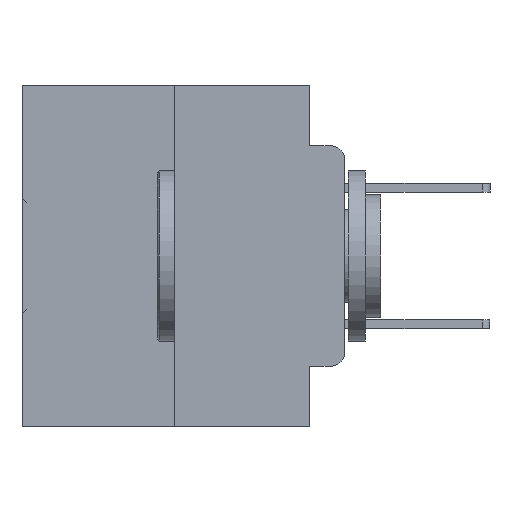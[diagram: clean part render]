
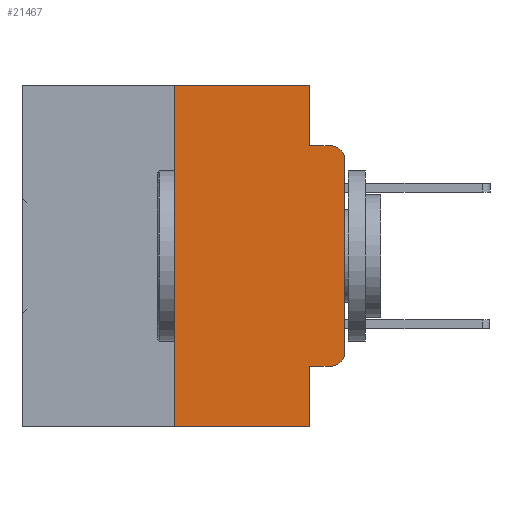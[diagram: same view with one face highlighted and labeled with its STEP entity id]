
A CAD part, left-side view. The second image highlights one B-rep face of the part: STEP entity #21467.
In plain terms, the highlighted planar face has unit normal (-1, 0, 0).
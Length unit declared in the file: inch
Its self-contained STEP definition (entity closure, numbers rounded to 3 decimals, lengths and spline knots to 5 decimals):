
#123 = EDGE_CURVE ( 'NONE', #16070, #5999, #28364, .T. ) ;
#210 = AXIS2_PLACEMENT_3D ( 'NONE', #16920, #19597, #10904 ) ;
#654 = DIRECTION ( 'NONE',  ( 0., 0., 1. ) ) ;
#675 = AXIS2_PLACEMENT_3D ( 'NONE', #14269, #32561, #16917 ) ;
#773 = AXIS2_PLACEMENT_3D ( 'NONE', #9756, #28203, #12435 ) ;
#1258 = EDGE_CURVE ( 'NONE', #7230, #16070, #28682, .T. ) ;
#2096 = DIRECTION ( 'NONE',  ( 0., -1., 0. ) ) ;
#2552 = DIRECTION ( 'NONE',  ( 0., 0., -1. ) ) ;
#2671 = CARTESIAN_POINT ( 'NONE',  ( 0., 0.051, -0.5 ) ) ;
#2820 = DIRECTION ( 'NONE',  ( 0., 0., 1. ) ) ;
#3560 = DIRECTION ( 'NONE',  ( 0., -1., 0. ) ) ;
#3790 = CARTESIAN_POINT ( 'NONE',  ( 0., 0.051, -0.0885 ) ) ;
#5045 = ORIENTED_EDGE ( 'NONE', *, *, #31380, .F. ) ;
#5073 = DIRECTION ( 'NONE',  ( 0., -1., 0. ) ) ;
#5190 = EDGE_CURVE ( 'NONE', #10859, #33024, #15728, .T. ) ;
#5338 = CARTESIAN_POINT ( 'NONE',  ( 0., 0., -0.3915 ) ) ;
#5439 = VERTEX_POINT ( 'NONE', #19984 ) ;
#5999 = VERTEX_POINT ( 'NONE', #5338 ) ;
#7084 = LINE ( 'NONE', #15355, #13293 ) ;
#7108 = CARTESIAN_POINT ( 'NONE',  ( 0., 0.25, -0.5 ) ) ;
#7230 = VERTEX_POINT ( 'NONE', #33657 ) ;
#7372 = EDGE_CURVE ( 'NONE', #12833, #12634, #31147, .T. ) ;
#7654 = VECTOR ( 'NONE', #11391, 39.37008 ) ;
#8013 = VECTOR ( 'NONE', #11854, 39.37008 ) ;
#9756 = CARTESIAN_POINT ( 'NONE',  ( 0., 0.02, -0.1085 ) ) ;
#10057 = ORIENTED_EDGE ( 'NONE', *, *, #17781, .F. ) ;
#10187 = VECTOR ( 'NONE', #2552, 39.37008 ) ;
#10456 = ORIENTED_EDGE ( 'NONE', *, *, #26624, .T. ) ;
#10742 = VECTOR ( 'NONE', #3560, 39.37008 ) ;
#10859 = VERTEX_POINT ( 'NONE', #7108 ) ;
#10904 = DIRECTION ( 'NONE',  ( 0., 0., -1. ) ) ;
#11391 = DIRECTION ( 'NONE',  ( 0., -1., 0. ) ) ;
#11719 = ORIENTED_EDGE ( 'NONE', *, *, #21932, .F. ) ;
#11854 = DIRECTION ( 'NONE',  ( 0., 0., -1. ) ) ;
#12435 = DIRECTION ( 'NONE',  ( 0., 0., -1. ) ) ;
#12529 = CARTESIAN_POINT ( 'NONE',  ( 0., 0.02, -0.4115 ) ) ;
#12634 = VERTEX_POINT ( 'NONE', #3790 ) ;
#12833 = VERTEX_POINT ( 'NONE', #25781 ) ;
#13293 = VECTOR ( 'NONE', #2096, 39.37008 ) ;
#13429 = CARTESIAN_POINT ( 'NONE',  ( 0., 0.25, 0. ) ) ;
#13781 = CARTESIAN_POINT ( 'NONE',  ( 0., 0.473, -0.5 ) ) ;
#14154 = CARTESIAN_POINT ( 'NONE',  ( 0., 0.473, 0. ) ) ;
#14269 = CARTESIAN_POINT ( 'NONE',  ( 0., 0.473, 0. ) ) ;
#15008 = ORIENTED_EDGE ( 'NONE', *, *, #27731, .T. ) ;
#15355 = CARTESIAN_POINT ( 'NONE',  ( 0., 0.051, -0.0885 ) ) ;
#15728 = LINE ( 'NONE', #13781, #22752 ) ;
#16070 = VERTEX_POINT ( 'NONE', #12529 ) ;
#16393 = LINE ( 'NONE', #19212, #29517 ) ;
#16912 = CIRCLE ( 'NONE', #773, 0.02 ) ;
#16917 = DIRECTION ( 'NONE',  ( 0., 0., -1. ) ) ;
#16920 = CARTESIAN_POINT ( 'NONE',  ( 0., 0.02, -0.3915 ) ) ;
#17060 = CARTESIAN_POINT ( 'NONE',  ( 0., 0.051, -0.4115 ) ) ;
#17781 = EDGE_CURVE ( 'NONE', #21798, #12833, #24795, .T. ) ;
#18148 = CARTESIAN_POINT ( 'NONE',  ( 0., 0.25, 0. ) ) ;
#18335 = ORIENTED_EDGE ( 'NONE', *, *, #1258, .T. ) ;
#19212 = CARTESIAN_POINT ( 'NONE',  ( 0., 0., 0. ) ) ;
#19597 = DIRECTION ( 'NONE',  ( -1., 0., 0. ) ) ;
#19685 = CARTESIAN_POINT ( 'NONE',  ( 0., 0.051, 0. ) ) ;
#19819 = VERTEX_POINT ( 'NONE', #23070 ) ;
#19984 = CARTESIAN_POINT ( 'NONE',  ( 0., 0., -0.1085 ) ) ;
#21467 = ADVANCED_FACE ( 'NONE', ( #31601 ), #22083, .F. ) ;
#21798 = VERTEX_POINT ( 'NONE', #18148 ) ;
#21932 = EDGE_CURVE ( 'NONE', #10859, #21798, #26320, .T. ) ;
#22039 = ORIENTED_EDGE ( 'NONE', *, *, #5190, .T. ) ;
#22083 = PLANE ( 'NONE',  #675 ) ;
#22752 = VECTOR ( 'NONE', #5073, 39.37008 ) ;
#23070 = CARTESIAN_POINT ( 'NONE',  ( 0., 0.02, -0.0885 ) ) ;
#23536 = EDGE_LOOP ( 'NONE', ( #15008, #10456, #5045, #28596, #10057, #11719, #22039, #30639, #18335, #33056 ) ) ;
#24795 = LINE ( 'NONE', #14154, #10742 ) ;
#25781 = CARTESIAN_POINT ( 'NONE',  ( 0., 0.051, 0. ) ) ;
#26320 = LINE ( 'NONE', #13429, #31571 ) ;
#26609 = LINE ( 'NONE', #19685, #8013 ) ;
#26624 = EDGE_CURVE ( 'NONE', #5439, #19819, #16912, .T. ) ;
#27731 = EDGE_CURVE ( 'NONE', #5999, #5439, #16393, .T. ) ;
#28203 = DIRECTION ( 'NONE',  ( -1., 0., 0. ) ) ;
#28364 = CIRCLE ( 'NONE', #210, 0.02 ) ;
#28596 = ORIENTED_EDGE ( 'NONE', *, *, #7372, .F. ) ;
#28682 = LINE ( 'NONE', #17060, #7654 ) ;
#29517 = VECTOR ( 'NONE', #654, 39.37008 ) ;
#29599 = EDGE_CURVE ( 'NONE', #7230, #33024, #26609, .T. ) ;
#30639 = ORIENTED_EDGE ( 'NONE', *, *, #29599, .F. ) ;
#31147 = LINE ( 'NONE', #31475, #10187 ) ;
#31380 = EDGE_CURVE ( 'NONE', #12634, #19819, #7084, .T. ) ;
#31475 = CARTESIAN_POINT ( 'NONE',  ( 0., 0.051, 0. ) ) ;
#31571 = VECTOR ( 'NONE', #2820, 39.37008 ) ;
#31601 = FACE_OUTER_BOUND ( 'NONE', #23536, .T. ) ;
#32561 = DIRECTION ( 'NONE',  ( 1., 0., 0. ) ) ;
#33024 = VERTEX_POINT ( 'NONE', #2671 ) ;
#33056 = ORIENTED_EDGE ( 'NONE', *, *, #123, .T. ) ;
#33657 = CARTESIAN_POINT ( 'NONE',  ( 0., 0.051, -0.4115 ) ) ;
